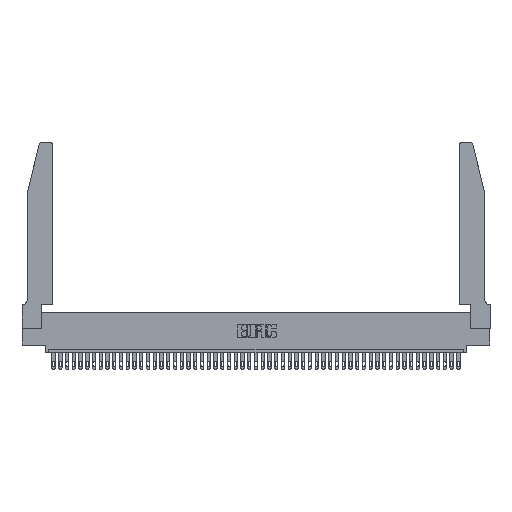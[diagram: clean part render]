
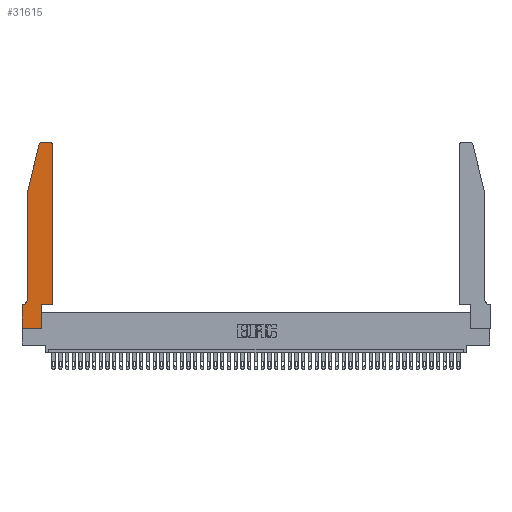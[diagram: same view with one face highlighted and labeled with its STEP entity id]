
A CAD part, top view. The second image highlights one B-rep face of the part: STEP entity #31615.
In plain terms, the highlighted planar face has unit normal (0, 0, 1).
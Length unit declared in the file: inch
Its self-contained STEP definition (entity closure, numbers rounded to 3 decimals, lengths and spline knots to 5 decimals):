
#319 = VERTEX_POINT ( 'NONE', #39305 ) ;
#422 = EDGE_CURVE ( 'NONE', #37351, #45128, #16871, .T. ) ;
#1319 = DIRECTION ( 'NONE',  ( 1., 0., 0. ) ) ;
#2812 = CARTESIAN_POINT ( 'NONE',  ( 0.4205, 2.75, 0.37 ) ) ;
#3100 = CARTESIAN_POINT ( 'NONE',  ( 0.2865, 0., 0.37 ) ) ;
#3650 = LINE ( 'NONE', #34266, #30993 ) ;
#3776 = CARTESIAN_POINT ( 'NONE',  ( 0.4505, 0.35, 0.37 ) ) ;
#4003 = VERTEX_POINT ( 'NONE', #9494 ) ;
#4407 = PLANE ( 'NONE',  #23000 ) ;
#5072 = DIRECTION ( 'NONE',  ( 0., 0., 1. ) ) ;
#6134 = VERTEX_POINT ( 'NONE', #19253 ) ;
#6928 = VECTOR ( 'NONE', #35927, 39.37008 ) ;
#6951 = VECTOR ( 'NONE', #15419, 39.37008 ) ;
#7464 = CARTESIAN_POINT ( 'NONE',  ( 0.0755, 2., 0.37 ) ) ;
#7670 = CARTESIAN_POINT ( 'NONE',  ( 0., 0., 0.37 ) ) ;
#7737 = EDGE_CURVE ( 'NONE', #11337, #39253, #37358, .T. ) ;
#7860 = CARTESIAN_POINT ( 'NONE',  ( 0.4505, 2.72, 0.37 ) ) ;
#8149 = ORIENTED_EDGE ( 'NONE', *, *, #45560, .T. ) ;
#8267 = DIRECTION ( 'NONE',  ( 0., 1., 0. ) ) ;
#8526 = DIRECTION ( 'NONE',  ( 0., 0., -1. ) ) ;
#8868 = FACE_OUTER_BOUND ( 'NONE', #25433, .T. ) ;
#9334 = CARTESIAN_POINT ( 'NONE',  ( 0., 0., 0.37 ) ) ;
#9494 = CARTESIAN_POINT ( 'NONE',  ( 0.284, 2.75, 0.37 ) ) ;
#10345 = VERTEX_POINT ( 'NONE', #3776 ) ;
#10642 = EDGE_CURVE ( 'NONE', #32842, #30733, #13344, .T. ) ;
#10947 = VECTOR ( 'NONE', #45439, 39.37008 ) ;
#11253 = CARTESIAN_POINT ( 'NONE',  ( 0.2865, 0.35, 0.37 ) ) ;
#11337 = VERTEX_POINT ( 'NONE', #9334 ) ;
#12282 = DIRECTION ( 'NONE',  ( -1., 0., 0. ) ) ;
#12594 = VECTOR ( 'NONE', #1319, 39.37008 ) ;
#12612 = CARTESIAN_POINT ( 'NONE',  ( 0.0055, 0.42, 0.37 ) ) ;
#13344 = CIRCLE ( 'NONE', #43826, 0.03 ) ;
#14057 = EDGE_CURVE ( 'NONE', #319, #11337, #25409, .T. ) ;
#14972 = LINE ( 'NONE', #34523, #12594 ) ;
#15200 = AXIS2_PLACEMENT_3D ( 'NONE', #12612, #8526, #12282 ) ;
#15225 = ORIENTED_EDGE ( 'NONE', *, *, #7737, .T. ) ;
#15313 = ORIENTED_EDGE ( 'NONE', *, *, #21241, .T. ) ;
#15419 = DIRECTION ( 'NONE',  ( -1., 0., 0. ) ) ;
#15762 = AXIS2_PLACEMENT_3D ( 'NONE', #25839, #32961, #18235 ) ;
#15887 = CARTESIAN_POINT ( 'NONE',  ( 0., 0.35, 0.37 ) ) ;
#15941 = CARTESIAN_POINT ( 'NONE',  ( 0.0755, 2., 0.37 ) ) ;
#16170 = LINE ( 'NONE', #44312, #33577 ) ;
#16677 = VECTOR ( 'NONE', #38637, 39.37008 ) ;
#16871 = LINE ( 'NONE', #24436, #6928 ) ;
#17649 = DIRECTION ( 'NONE',  ( 1., 0., 0. ) ) ;
#18235 = DIRECTION ( 'NONE',  ( 1., 0., 0. ) ) ;
#19159 = CARTESIAN_POINT ( 'NONE',  ( 0.0755, 0.35, 0.37 ) ) ;
#19253 = CARTESIAN_POINT ( 'NONE',  ( 0.2865, 0.35, 0.37 ) ) ;
#19458 = ORIENTED_EDGE ( 'NONE', *, *, #44264, .T. ) ;
#19673 = CARTESIAN_POINT ( 'NONE',  ( 0.25487, 2.72718, 0.37 ) ) ;
#19794 = CIRCLE ( 'NONE', #15762, 0.03 ) ;
#19967 = LINE ( 'NONE', #11253, #20597 ) ;
#20597 = VECTOR ( 'NONE', #25760, 39.37008 ) ;
#21241 = EDGE_CURVE ( 'NONE', #45128, #33732, #45973, .T. ) ;
#21338 = CARTESIAN_POINT ( 'NONE',  ( 0., 0., 0.37 ) ) ;
#21831 = DIRECTION ( 'NONE',  ( 0., 0., 1. ) ) ;
#23000 = AXIS2_PLACEMENT_3D ( 'NONE', #15887, #5072, #30621 ) ;
#24436 = CARTESIAN_POINT ( 'NONE',  ( 0.0755, 2., 0.37 ) ) ;
#25409 = LINE ( 'NONE', #7670, #16677 ) ;
#25433 = EDGE_LOOP ( 'NONE', ( #32802, #19458, #8149, #33810, #15313, #33481, #26747, #15225, #46889, #45867, #38832, #46509 ) ) ;
#25567 = VERTEX_POINT ( 'NONE', #19673 ) ;
#25760 = DIRECTION ( 'NONE',  ( 0., 1., 0. ) ) ;
#25839 = CARTESIAN_POINT ( 'NONE',  ( 0.284, 2.72, 0.37 ) ) ;
#26016 = DIRECTION ( 'NONE',  ( -1., 0., 0. ) ) ;
#26359 = CARTESIAN_POINT ( 'NONE',  ( 0.4205, 2.72, 0.37 ) ) ;
#26747 = ORIENTED_EDGE ( 'NONE', *, *, #14057, .T. ) ;
#29756 = EDGE_CURVE ( 'NONE', #39253, #6134, #19967, .T. ) ;
#30621 = DIRECTION ( 'NONE',  ( 1., 0., 0. ) ) ;
#30733 = VERTEX_POINT ( 'NONE', #2812 ) ;
#30990 = VECTOR ( 'NONE', #42856, 39.37008 ) ;
#30993 = VECTOR ( 'NONE', #8267, 39.37008 ) ;
#31615 = ADVANCED_FACE ( 'NONE', ( #8868 ), #4407, .T. ) ;
#32802 = ORIENTED_EDGE ( 'NONE', *, *, #40040, .T. ) ;
#32842 = VERTEX_POINT ( 'NONE', #7860 ) ;
#32961 = DIRECTION ( 'NONE',  ( 0., 0., 1. ) ) ;
#33481 = ORIENTED_EDGE ( 'NONE', *, *, #34049, .T. ) ;
#33577 = VECTOR ( 'NONE', #26016, 39.37008 ) ;
#33732 = VERTEX_POINT ( 'NONE', #43014 ) ;
#33810 = ORIENTED_EDGE ( 'NONE', *, *, #422, .T. ) ;
#34049 = EDGE_CURVE ( 'NONE', #33732, #319, #40611, .T. ) ;
#34266 = CARTESIAN_POINT ( 'NONE',  ( 0.4505, 0.35, 0.37 ) ) ;
#34523 = CARTESIAN_POINT ( 'NONE',  ( 0.4505, 0.35, 0.37 ) ) ;
#35927 = DIRECTION ( 'NONE',  ( 0., -1., 0. ) ) ;
#37351 = VERTEX_POINT ( 'NONE', #7464 ) ;
#37358 = LINE ( 'NONE', #21338, #30990 ) ;
#38637 = DIRECTION ( 'NONE',  ( 0., -1., 0. ) ) ;
#38832 = ORIENTED_EDGE ( 'NONE', *, *, #41983, .T. ) ;
#39253 = VERTEX_POINT ( 'NONE', #3100 ) ;
#39305 = CARTESIAN_POINT ( 'NONE',  ( 0., 0.35, 0.37 ) ) ;
#40040 = EDGE_CURVE ( 'NONE', #30733, #4003, #16170, .T. ) ;
#40611 = LINE ( 'NONE', #19159, #6951 ) ;
#41983 = EDGE_CURVE ( 'NONE', #10345, #32842, #3650, .T. ) ;
#42856 = DIRECTION ( 'NONE',  ( 1., 0., 0. ) ) ;
#43014 = CARTESIAN_POINT ( 'NONE',  ( 0.0055, 0.35, 0.37 ) ) ;
#43826 = AXIS2_PLACEMENT_3D ( 'NONE', #26359, #21831, #17649 ) ;
#44264 = EDGE_CURVE ( 'NONE', #4003, #25567, #19794, .T. ) ;
#44312 = CARTESIAN_POINT ( 'NONE',  ( 0.2605, 2.75, 0.37 ) ) ;
#45128 = VERTEX_POINT ( 'NONE', #46827 ) ;
#45439 = DIRECTION ( 'NONE',  ( -0.239, -0.971, 0. ) ) ;
#45560 = EDGE_CURVE ( 'NONE', #25567, #37351, #46369, .T. ) ;
#45867 = ORIENTED_EDGE ( 'NONE', *, *, #46224, .T. ) ;
#45973 = CIRCLE ( 'NONE', #15200, 0.07 ) ;
#46224 = EDGE_CURVE ( 'NONE', #6134, #10345, #14972, .T. ) ;
#46369 = LINE ( 'NONE', #15941, #10947 ) ;
#46509 = ORIENTED_EDGE ( 'NONE', *, *, #10642, .T. ) ;
#46827 = CARTESIAN_POINT ( 'NONE',  ( 0.0755, 0.42, 0.37 ) ) ;
#46889 = ORIENTED_EDGE ( 'NONE', *, *, #29756, .T. ) ;
